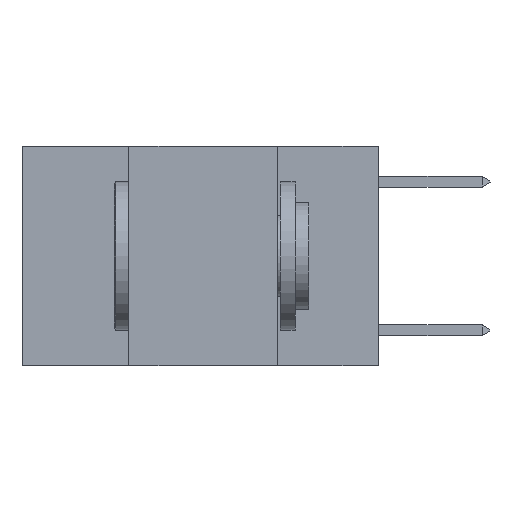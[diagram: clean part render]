
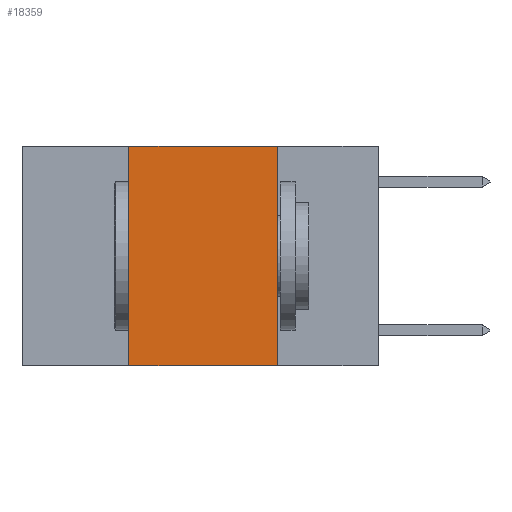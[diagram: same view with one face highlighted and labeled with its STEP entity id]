
A CAD part, left-side view. The second image highlights one B-rep face of the part: STEP entity #18359.
In plain terms, the highlighted planar face has unit normal (-1, 0, 0).
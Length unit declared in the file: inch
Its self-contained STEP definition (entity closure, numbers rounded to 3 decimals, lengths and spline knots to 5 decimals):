
#55 = VERTEX_POINT ( 'NONE', #1475 ) ;
#1409 = DIRECTION ( 'NONE',  ( 0., 0., -1. ) ) ;
#1475 = CARTESIAN_POINT ( 'NONE',  ( 0., 0.42, -0.37 ) ) ;
#1801 = ORIENTED_EDGE ( 'NONE', *, *, #17771, .F. ) ;
#3191 = PLANE ( 'NONE',  #23536 ) ;
#3316 = DIRECTION ( 'NONE',  ( 1., 0., 0. ) ) ;
#3338 = LINE ( 'NONE', #10707, #16241 ) ;
#5815 = VECTOR ( 'NONE', #13379, 39.37008 ) ;
#6029 = LINE ( 'NONE', #9727, #21852 ) ;
#6069 = CARTESIAN_POINT ( 'NONE',  ( 0., 0.17, 0. ) ) ;
#7174 = EDGE_CURVE ( 'NONE', #55, #20605, #6029, .T. ) ;
#8694 = CARTESIAN_POINT ( 'NONE',  ( 0., 0.17, 0. ) ) ;
#8746 = VECTOR ( 'NONE', #21447, 39.37008 ) ;
#9349 = LINE ( 'NONE', #16606, #5815 ) ;
#9727 = CARTESIAN_POINT ( 'NONE',  ( 0., 0.42, 0. ) ) ;
#9779 = ORIENTED_EDGE ( 'NONE', *, *, #21553, .F. ) ;
#10458 = CARTESIAN_POINT ( 'NONE',  ( 0., 0.6, 0. ) ) ;
#10459 = LINE ( 'NONE', #8694, #8746 ) ;
#10707 = CARTESIAN_POINT ( 'NONE',  ( 0., 0.6, 0. ) ) ;
#10767 = EDGE_CURVE ( 'NONE', #55, #12463, #9349, .T. ) ;
#12463 = VERTEX_POINT ( 'NONE', #16093 ) ;
#13379 = DIRECTION ( 'NONE',  ( 0., -1., 0. ) ) ;
#16093 = CARTESIAN_POINT ( 'NONE',  ( 0., 0.17, -0.37 ) ) ;
#16241 = VECTOR ( 'NONE', #17864, 39.37008 ) ;
#16606 = CARTESIAN_POINT ( 'NONE',  ( 0., 0.6, -0.37 ) ) ;
#17771 = EDGE_CURVE ( 'NONE', #20605, #21734, #3338, .T. ) ;
#17864 = DIRECTION ( 'NONE',  ( 0., -1., 0. ) ) ;
#18359 = ADVANCED_FACE ( 'NONE', ( #19520 ), #3191, .F. ) ;
#18804 = CARTESIAN_POINT ( 'NONE',  ( 0., 0.42, 0. ) ) ;
#18895 = DIRECTION ( 'NONE',  ( 0., 0., 1. ) ) ;
#19089 = EDGE_LOOP ( 'NONE', ( #9779, #1801, #20455, #20368 ) ) ;
#19520 = FACE_OUTER_BOUND ( 'NONE', #19089, .T. ) ;
#20368 = ORIENTED_EDGE ( 'NONE', *, *, #10767, .T. ) ;
#20455 = ORIENTED_EDGE ( 'NONE', *, *, #7174, .F. ) ;
#20605 = VERTEX_POINT ( 'NONE', #18804 ) ;
#21447 = DIRECTION ( 'NONE',  ( 0., 0., -1. ) ) ;
#21553 = EDGE_CURVE ( 'NONE', #21734, #12463, #10459, .T. ) ;
#21734 = VERTEX_POINT ( 'NONE', #6069 ) ;
#21852 = VECTOR ( 'NONE', #18895, 39.37008 ) ;
#23536 = AXIS2_PLACEMENT_3D ( 'NONE', #10458, #3316, #1409 ) ;
